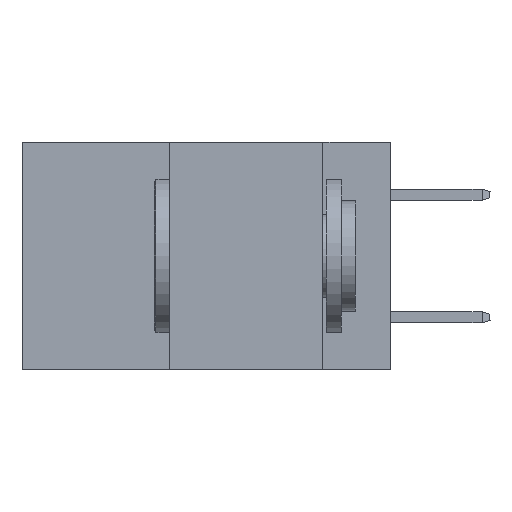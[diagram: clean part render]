
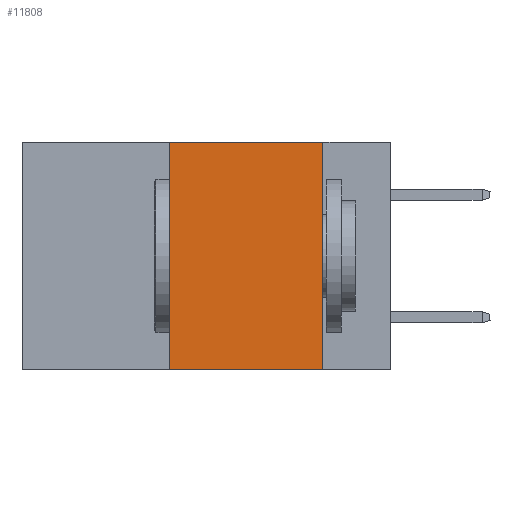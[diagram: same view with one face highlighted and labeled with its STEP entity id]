
A CAD part, left-side view. The second image highlights one B-rep face of the part: STEP entity #11808.
In plain terms, the highlighted planar face has unit normal (-1, 0, 0).
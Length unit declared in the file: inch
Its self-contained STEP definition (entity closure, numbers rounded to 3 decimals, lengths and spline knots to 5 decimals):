
#1382 = DIRECTION ( 'NONE',  ( 0., 0., -1. ) ) ;
#2259 = EDGE_CURVE ( 'NONE', #29273, #18333, #12444, .T. ) ;
#2434 = DIRECTION ( 'NONE',  ( 0., -1., 0. ) ) ;
#2558 = ORIENTED_EDGE ( 'NONE', *, *, #9897, .F. ) ;
#3549 = DIRECTION ( 'NONE',  ( 0., 0., 1. ) ) ;
#5775 = VECTOR ( 'NONE', #3549, 39.37008 ) ;
#6818 = CARTESIAN_POINT ( 'NONE',  ( 0., 0.11, 0. ) ) ;
#7232 = DIRECTION ( 'NONE',  ( 0., 0., -1. ) ) ;
#7443 = CARTESIAN_POINT ( 'NONE',  ( 0., 0.11, -0.37 ) ) ;
#9473 = PLANE ( 'NONE',  #13709 ) ;
#9897 = EDGE_CURVE ( 'NONE', #18333, #13443, #26727, .T. ) ;
#10873 = FACE_OUTER_BOUND ( 'NONE', #23446, .T. ) ;
#10986 = VERTEX_POINT ( 'NONE', #19566 ) ;
#11808 = ADVANCED_FACE ( 'NONE', ( #10873 ), #9473, .F. ) ;
#11946 = CARTESIAN_POINT ( 'NONE',  ( 0., 0.36, 0. ) ) ;
#12444 = LINE ( 'NONE', #25544, #34843 ) ;
#12853 = CARTESIAN_POINT ( 'NONE',  ( 0., 0.11, 0. ) ) ;
#12987 = ORIENTED_EDGE ( 'NONE', *, *, #26254, .T. ) ;
#13443 = VERTEX_POINT ( 'NONE', #7443 ) ;
#13709 = AXIS2_PLACEMENT_3D ( 'NONE', #15580, #21757, #7232 ) ;
#13931 = ORIENTED_EDGE ( 'NONE', *, *, #2259, .F. ) ;
#15303 = LINE ( 'NONE', #36752, #29263 ) ;
#15580 = CARTESIAN_POINT ( 'NONE',  ( 0., 0.6, 0. ) ) ;
#17059 = CARTESIAN_POINT ( 'NONE',  ( 0., 0.36, 0. ) ) ;
#18333 = VERTEX_POINT ( 'NONE', #12853 ) ;
#19121 = VECTOR ( 'NONE', #1382, 39.37008 ) ;
#19566 = CARTESIAN_POINT ( 'NONE',  ( 0., 0.36, -0.37 ) ) ;
#21757 = DIRECTION ( 'NONE',  ( 1., 0., 0. ) ) ;
#23446 = EDGE_LOOP ( 'NONE', ( #2558, #13931, #32994, #12987 ) ) ;
#25299 = DIRECTION ( 'NONE',  ( 0., -1., 0. ) ) ;
#25498 = LINE ( 'NONE', #11946, #5775 ) ;
#25544 = CARTESIAN_POINT ( 'NONE',  ( 0., 0.6, 0. ) ) ;
#26254 = EDGE_CURVE ( 'NONE', #10986, #13443, #15303, .T. ) ;
#26727 = LINE ( 'NONE', #6818, #19121 ) ;
#29263 = VECTOR ( 'NONE', #2434, 39.37008 ) ;
#29273 = VERTEX_POINT ( 'NONE', #17059 ) ;
#32430 = EDGE_CURVE ( 'NONE', #10986, #29273, #25498, .T. ) ;
#32994 = ORIENTED_EDGE ( 'NONE', *, *, #32430, .F. ) ;
#34843 = VECTOR ( 'NONE', #25299, 39.37008 ) ;
#36752 = CARTESIAN_POINT ( 'NONE',  ( 0., 0.6, -0.37 ) ) ;
